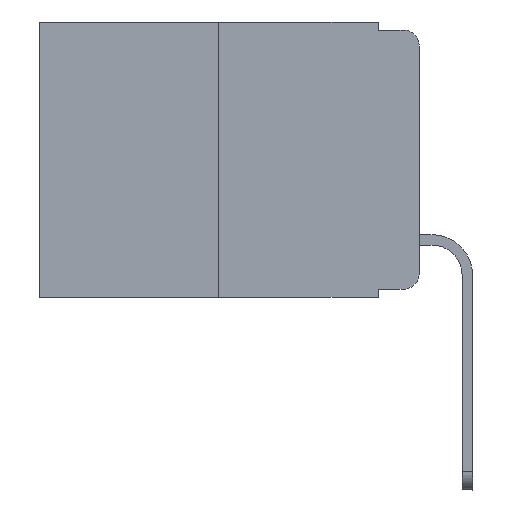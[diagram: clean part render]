
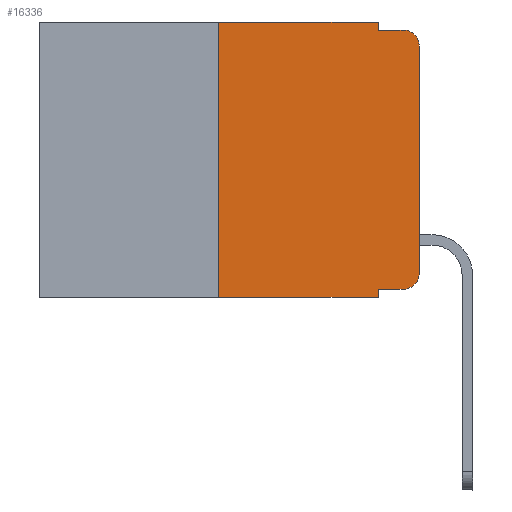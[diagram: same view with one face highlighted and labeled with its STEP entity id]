
A CAD part, left-side view. The second image highlights one B-rep face of the part: STEP entity #16336.
In plain terms, the highlighted planar face has unit normal (-1, 0, 0).
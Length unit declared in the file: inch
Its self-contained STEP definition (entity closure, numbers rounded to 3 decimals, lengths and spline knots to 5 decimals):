
#114 = EDGE_CURVE ( 'NONE', #7022, #12088, #9708, .T. ) ;
#125 = ORIENTED_EDGE ( 'NONE', *, *, #7106, .F. ) ;
#1022 = DIRECTION ( 'NONE',  ( 0., 0., 1. ) ) ;
#1252 = CARTESIAN_POINT ( 'NONE',  ( 0., 0.051, 0. ) ) ;
#1403 = VERTEX_POINT ( 'NONE', #16702 ) ;
#2227 = CARTESIAN_POINT ( 'NONE',  ( 0., 0.02, -0.03 ) ) ;
#2420 = EDGE_CURVE ( 'NONE', #6076, #12649, #4715, .T. ) ;
#2445 = VECTOR ( 'NONE', #13688, 39.37008 ) ;
#2455 = CARTESIAN_POINT ( 'NONE',  ( 0., 0.473, 0. ) ) ;
#2457 = LINE ( 'NONE', #2797, #2445 ) ;
#2797 = CARTESIAN_POINT ( 'NONE',  ( 0., 0.051, -0.333 ) ) ;
#2945 = VECTOR ( 'NONE', #1022, 39.37008 ) ;
#3323 = ORIENTED_EDGE ( 'NONE', *, *, #4603, .F. ) ;
#3347 = VECTOR ( 'NONE', #16225, 39.37008 ) ;
#3505 = ORIENTED_EDGE ( 'NONE', *, *, #16051, .T. ) ;
#3834 = VECTOR ( 'NONE', #12006, 39.37008 ) ;
#4028 = CARTESIAN_POINT ( 'NONE',  ( 0., 0.051, -0.01 ) ) ;
#4603 = EDGE_CURVE ( 'NONE', #8677, #5565, #14941, .T. ) ;
#4715 = CIRCLE ( 'NONE', #12209, 0.02 ) ;
#4730 = DIRECTION ( 'NONE',  ( 0., 0., -1. ) ) ;
#5096 = CARTESIAN_POINT ( 'NONE',  ( 0., 0.051, -0.333 ) ) ;
#5160 = FACE_OUTER_BOUND ( 'NONE', #12451, .T. ) ;
#5229 = CARTESIAN_POINT ( 'NONE',  ( 0., 0., 0. ) ) ;
#5565 = VERTEX_POINT ( 'NONE', #1252 ) ;
#5788 = CARTESIAN_POINT ( 'NONE',  ( 0., 0.25, 0. ) ) ;
#5883 = CARTESIAN_POINT ( 'NONE',  ( 0., 0.051, 0. ) ) ;
#6076 = VERTEX_POINT ( 'NONE', #8304 ) ;
#6138 = CARTESIAN_POINT ( 'NONE',  ( 0., 0.02, -0.01 ) ) ;
#6397 = AXIS2_PLACEMENT_3D ( 'NONE', #2227, #7690, #17234 ) ;
#6874 = VERTEX_POINT ( 'NONE', #5096 ) ;
#7022 = VERTEX_POINT ( 'NONE', #16434 ) ;
#7106 = EDGE_CURVE ( 'NONE', #6874, #7602, #12748, .T. ) ;
#7240 = EDGE_CURVE ( 'NONE', #1403, #12088, #13312, .T. ) ;
#7515 = EDGE_CURVE ( 'NONE', #5565, #7022, #10216, .T. ) ;
#7602 = VERTEX_POINT ( 'NONE', #7847 ) ;
#7690 = DIRECTION ( 'NONE',  ( -1., 0., 0. ) ) ;
#7825 = CARTESIAN_POINT ( 'NONE',  ( 0., 0.25, 0. ) ) ;
#7847 = CARTESIAN_POINT ( 'NONE',  ( 0., 0.051, -0.343 ) ) ;
#8096 = EDGE_CURVE ( 'NONE', #15661, #8677, #13068, .T. ) ;
#8110 = LINE ( 'NONE', #5229, #3347 ) ;
#8304 = CARTESIAN_POINT ( 'NONE',  ( 0., 0.02, -0.333 ) ) ;
#8433 = VECTOR ( 'NONE', #15688, 39.37008 ) ;
#8677 = VERTEX_POINT ( 'NONE', #5788 ) ;
#8846 = DIRECTION ( 'NONE',  ( -1., 0., 0. ) ) ;
#9233 = PLANE ( 'NONE',  #16356 ) ;
#9249 = CARTESIAN_POINT ( 'NONE',  ( 0., 0.473, -0.343 ) ) ;
#9473 = EDGE_CURVE ( 'NONE', #6874, #6076, #2457, .T. ) ;
#9708 = LINE ( 'NONE', #4028, #11454 ) ;
#10216 = LINE ( 'NONE', #11659, #8433 ) ;
#10307 = ORIENTED_EDGE ( 'NONE', *, *, #114, .F. ) ;
#10415 = DIRECTION ( 'NONE',  ( 1., 0., 0. ) ) ;
#10450 = ORIENTED_EDGE ( 'NONE', *, *, #9473, .T. ) ;
#10504 = CARTESIAN_POINT ( 'NONE',  ( 0., 0.473, 0. ) ) ;
#10718 = EDGE_CURVE ( 'NONE', #12649, #1403, #8110, .T. ) ;
#10967 = DIRECTION ( 'NONE',  ( 0., -1., 0. ) ) ;
#11454 = VECTOR ( 'NONE', #10967, 39.37008 ) ;
#11557 = ORIENTED_EDGE ( 'NONE', *, *, #2420, .T. ) ;
#11659 = CARTESIAN_POINT ( 'NONE',  ( 0., 0.051, 0. ) ) ;
#12006 = DIRECTION ( 'NONE',  ( 0., -1., 0. ) ) ;
#12088 = VERTEX_POINT ( 'NONE', #6138 ) ;
#12209 = AXIS2_PLACEMENT_3D ( 'NONE', #15763, #8846, #17109 ) ;
#12451 = EDGE_LOOP ( 'NONE', ( #14744, #12986, #10307, #15073, #3323, #16563, #3505, #125, #10450, #11557 ) ) ;
#12649 = VERTEX_POINT ( 'NONE', #15828 ) ;
#12748 = LINE ( 'NONE', #5883, #14090 ) ;
#12986 = ORIENTED_EDGE ( 'NONE', *, *, #7240, .T. ) ;
#13068 = LINE ( 'NONE', #7825, #2945 ) ;
#13120 = DIRECTION ( 'NONE',  ( 0., -1., 0. ) ) ;
#13193 = DIRECTION ( 'NONE',  ( 0., 0., -1. ) ) ;
#13312 = CIRCLE ( 'NONE', #6397, 0.02 ) ;
#13688 = DIRECTION ( 'NONE',  ( 0., -1., 0. ) ) ;
#14090 = VECTOR ( 'NONE', #4730, 39.37008 ) ;
#14464 = LINE ( 'NONE', #9249, #15194 ) ;
#14744 = ORIENTED_EDGE ( 'NONE', *, *, #10718, .T. ) ;
#14941 = LINE ( 'NONE', #2455, #3834 ) ;
#15073 = ORIENTED_EDGE ( 'NONE', *, *, #7515, .F. ) ;
#15194 = VECTOR ( 'NONE', #13120, 39.37008 ) ;
#15661 = VERTEX_POINT ( 'NONE', #17618 ) ;
#15688 = DIRECTION ( 'NONE',  ( 0., 0., -1. ) ) ;
#15763 = CARTESIAN_POINT ( 'NONE',  ( 0., 0.02, -0.313 ) ) ;
#15828 = CARTESIAN_POINT ( 'NONE',  ( 0., 0., -0.313 ) ) ;
#16051 = EDGE_CURVE ( 'NONE', #15661, #7602, #14464, .T. ) ;
#16225 = DIRECTION ( 'NONE',  ( 0., 0., 1. ) ) ;
#16336 = ADVANCED_FACE ( 'NONE', ( #5160 ), #9233, .F. ) ;
#16356 = AXIS2_PLACEMENT_3D ( 'NONE', #10504, #10415, #13193 ) ;
#16434 = CARTESIAN_POINT ( 'NONE',  ( 0., 0.051, -0.01 ) ) ;
#16563 = ORIENTED_EDGE ( 'NONE', *, *, #8096, .F. ) ;
#16702 = CARTESIAN_POINT ( 'NONE',  ( 0., 0., -0.03 ) ) ;
#17109 = DIRECTION ( 'NONE',  ( 0., 0., -1. ) ) ;
#17234 = DIRECTION ( 'NONE',  ( 0., 0., -1. ) ) ;
#17618 = CARTESIAN_POINT ( 'NONE',  ( 0., 0.25, -0.343 ) ) ;
